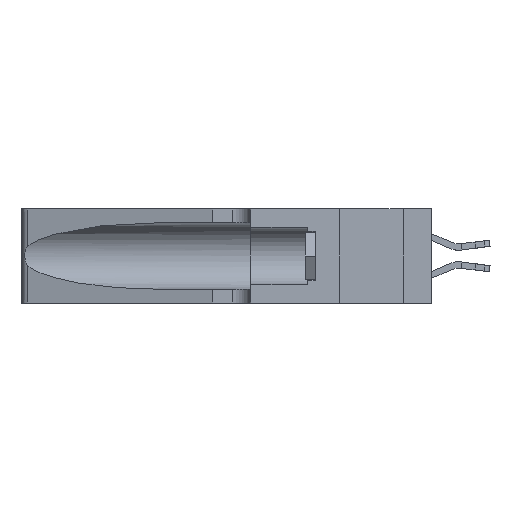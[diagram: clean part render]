
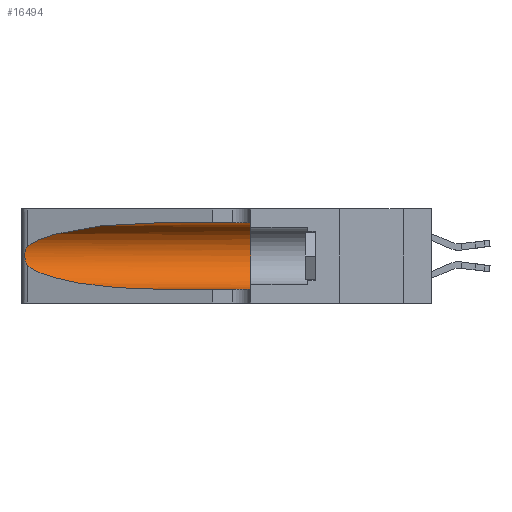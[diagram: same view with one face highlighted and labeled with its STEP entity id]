
A CAD part, left-side view. The second image highlights one B-rep face of the part: STEP entity #16494.
In plain terms, the highlighted cylindrical face has radius 3.308 mm (diameter 6.617 mm), a partial arc.
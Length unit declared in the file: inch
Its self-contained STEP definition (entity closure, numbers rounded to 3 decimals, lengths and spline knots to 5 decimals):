
#290 = CARTESIAN_POINT ( 'NONE',  ( 0.25639, 1.23186, 0.15144 ) ) ;
#681 = ORIENTED_EDGE ( 'NONE', *, *, #9678, .F. ) ;
#720 = CARTESIAN_POINT ( 'NONE',  ( 0.2373, 1.15595, 0.28018 ) ) ;
#2468 = DIRECTION ( 'NONE',  ( 0., 1., 0. ) ) ;
#2803 = CARTESIAN_POINT ( 'NONE',  ( 0.1305, 0.35, 0.05475 ) ) ;
#3126 = CARTESIAN_POINT ( 'NONE',  ( 0.25487, 1.22718, 0.14631 ) ) ;
#3254 = CARTESIAN_POINT ( 'NONE',  ( 0.25487, 1.22718, 0.14631 ) ) ;
#5512 = VERTEX_POINT ( 'NONE', #2803 ) ;
#5831 = CARTESIAN_POINT ( 'NONE',  ( 0.25639, 1.23184, 0.21858 ) ) ;
#6042 = VECTOR ( 'NONE', #17590, 39.37008 ) ;
#6077 = CARTESIAN_POINT ( 'NONE',  ( 0.1305, 0.35, 0.31525 ) ) ;
#6101 = CARTESIAN_POINT ( 'NONE',  ( 0.2373, 1.15595, 0.08982 ) ) ;
#8093 = CARTESIAN_POINT ( 'NONE',  ( 0.1305, 0.72297, 0.05475 ) ) ;
#8285 = EDGE_LOOP ( 'NONE', ( #33692, #34005, #19874, #8455, #10150, #681 ) ) ;
#8455 = ORIENTED_EDGE ( 'NONE', *, *, #14451, .T. ) ;
#8615 = CARTESIAN_POINT ( 'NONE',  ( 0.25854, 1.2359, 0.20912 ) ) ;
#8870 = CARTESIAN_POINT ( 'NONE',  ( 0.1305, 0.72297, 0.05475 ) ) ;
#9459 = VERTEX_POINT ( 'NONE', #14074 ) ;
#9678 = EDGE_CURVE ( 'NONE', #25126, #32084, #20475, .T. ) ;
#10150 = ORIENTED_EDGE ( 'NONE', *, *, #31364, .F. ) ;
#11376 = CARTESIAN_POINT ( 'NONE',  ( 0.26075, 1.23896, 0.19203 ) ) ;
#13995 = CARTESIAN_POINT ( 'NONE',  ( 0.25555, 1.22994, 0.2215 ) ) ;
#14074 = CARTESIAN_POINT ( 'NONE',  ( 0.25487, 1.22718, 0.22369 ) ) ;
#14109 = CARTESIAN_POINT ( 'NONE',  ( 0.26017, 1.23833, 0.17102 ) ) ;
#14134 = AXIS2_PLACEMENT_3D ( 'NONE', #18867, #2468, #21555 ) ;
#14331 = FACE_OUTER_BOUND ( 'NONE', #8285, .T. ) ;
#14451 = EDGE_CURVE ( 'NONE', #16416, #5512, #34592, .T. ) ;
#14799 =( BOUNDED_CURVE ( )  B_SPLINE_CURVE ( 3, ( #17227, #33054, #720, #19912 ),
 .UNSPECIFIED., .F., .T. ) 
 B_SPLINE_CURVE_WITH_KNOTS ( ( 4, 4 ),
 ( 1.5708, 2.84003 ),
 .UNSPECIFIED. ) 
 CURVE ( )  GEOMETRIC_REPRESENTATION_ITEM ( )  RATIONAL_B_SPLINE_CURVE ( ( 1., 0.87, 0.87, 1. ) ) 
 REPRESENTATION_ITEM ( '' )  );
#14902 = CARTESIAN_POINT ( 'NONE',  ( 0.1305, 1.61858, 0.31525 ) ) ;
#16416 = VERTEX_POINT ( 'NONE', #8093 ) ;
#16494 = ADVANCED_FACE ( 'NONE', ( #14331 ), #20605, .F. ) ;
#16692 = CARTESIAN_POINT ( 'NONE',  ( 0.25487, 1.22718, 0.22369 ) ) ;
#16812 = CARTESIAN_POINT ( 'NONE',  ( 0.25789, 1.23486, 0.15765 ) ) ;
#17227 = CARTESIAN_POINT ( 'NONE',  ( 0.1305, 0.72297, 0.31525 ) ) ;
#17590 = DIRECTION ( 'NONE',  ( 0., -1., 0. ) ) ;
#18408 =( BOUNDED_CURVE ( )  B_SPLINE_CURVE ( 3, ( #3254, #6101, #24961, #8870 ),
 .UNSPECIFIED., .F., .F. ) 
 B_SPLINE_CURVE_WITH_KNOTS ( ( 4, 4 ),
 ( 3.44316, 4.71239 ),
 .UNSPECIFIED. ) 
 CURVE ( )  GEOMETRIC_REPRESENTATION_ITEM ( )  RATIONAL_B_SPLINE_CURVE ( ( 1., 0.87, 0.87, 1. ) ) 
 REPRESENTATION_ITEM ( '' )  );
#18867 = CARTESIAN_POINT ( 'NONE',  ( 0.1305, 0.35, 0.185 ) ) ;
#19117 = DIRECTION ( 'NONE',  ( 0., -1., 0. ) ) ;
#19503 = CARTESIAN_POINT ( 'NONE',  ( 0.25555, 1.22993, 0.14849 ) ) ;
#19710 = VERTEX_POINT ( 'NONE', #21700 ) ;
#19874 = ORIENTED_EDGE ( 'NONE', *, *, #30316, .T. ) ;
#19912 = CARTESIAN_POINT ( 'NONE',  ( 0.25487, 1.22718, 0.22369 ) ) ;
#20475 = LINE ( 'NONE', #14902, #6042 ) ;
#20605 = CYLINDRICAL_SURFACE ( 'NONE', #20803, 0.13025 ) ;
#20803 = AXIS2_PLACEMENT_3D ( 'NONE', #24460, #19117, #34930 ) ;
#21555 = DIRECTION ( 'NONE',  ( 0., 0., 1. ) ) ;
#21700 = CARTESIAN_POINT ( 'NONE',  ( 0.25487, 1.22718, 0.14631 ) ) ;
#22431 = CARTESIAN_POINT ( 'NONE',  ( 0.1305, 0.72297, 0.31525 ) ) ;
#22488 = EDGE_CURVE ( 'NONE', #25126, #9459, #14799, .T. ) ;
#23880 = CARTESIAN_POINT ( 'NONE',  ( 0.1305, 1.61858, 0.05475 ) ) ;
#24388 = CIRCLE ( 'NONE', #14134, 0.13025 ) ;
#24460 = CARTESIAN_POINT ( 'NONE',  ( 0.1305, 1.61858, 0.185 ) ) ;
#24723 = CARTESIAN_POINT ( 'NONE',  ( 0.25787, 1.23484, 0.2124 ) ) ;
#24961 = CARTESIAN_POINT ( 'NONE',  ( 0.18966, 0.96281, 0.05475 ) ) ;
#25126 = VERTEX_POINT ( 'NONE', #22431 ) ;
#27380 = CARTESIAN_POINT ( 'NONE',  ( 0.26018, 1.23835, 0.19895 ) ) ;
#27624 = VECTOR ( 'NONE', #34445, 39.37008 ) ;
#30023 = CARTESIAN_POINT ( 'NONE',  ( 0.26075, 1.23896, 0.178 ) ) ;
#30316 = EDGE_CURVE ( 'NONE', #19710, #16416, #18408, .T. ) ;
#31364 = EDGE_CURVE ( 'NONE', #32084, #5512, #24388, .T. ) ;
#32084 = VERTEX_POINT ( 'NONE', #6077 ) ;
#32643 = CARTESIAN_POINT ( 'NONE',  ( 0.25856, 1.23593, 0.16098 ) ) ;
#33054 = CARTESIAN_POINT ( 'NONE',  ( 0.18966, 0.96281, 0.31525 ) ) ;
#33692 = ORIENTED_EDGE ( 'NONE', *, *, #22488, .T. ) ;
#33904 = EDGE_CURVE ( 'NONE', #9459, #19710, #34291, .T. ) ;
#34005 = ORIENTED_EDGE ( 'NONE', *, *, #33904, .T. ) ;
#34291 = B_SPLINE_CURVE_WITH_KNOTS ( 'NONE', 3,
 ( #16692, #13995, #5831, #24723, #8615, #27380, #11376, #30023, #14109, #32643, #16812, #290, #19503, #3126 ),
 .UNSPECIFIED., .F., .F.,
 ( 4, 2, 2, 2, 2, 2, 4 ),
 ( 0., 0.00027, 0.00053, 0.00107, 0.0016, 0.00187, 0.00214 ),
 .UNSPECIFIED. ) ;
#34445 = DIRECTION ( 'NONE',  ( 0., -1., 0. ) ) ;
#34592 = LINE ( 'NONE', #23880, #27624 ) ;
#34930 = DIRECTION ( 'NONE',  ( 0., 0., -1. ) ) ;
